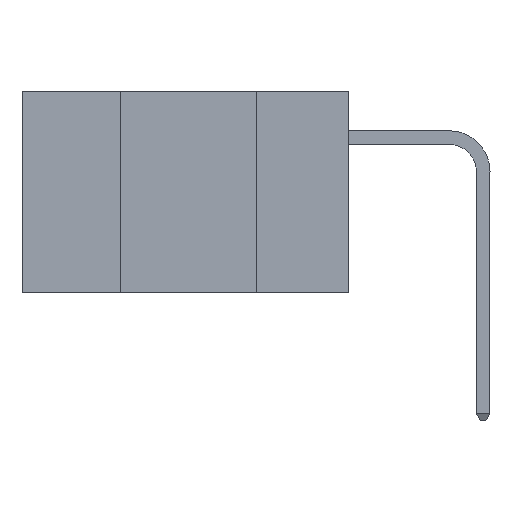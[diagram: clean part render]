
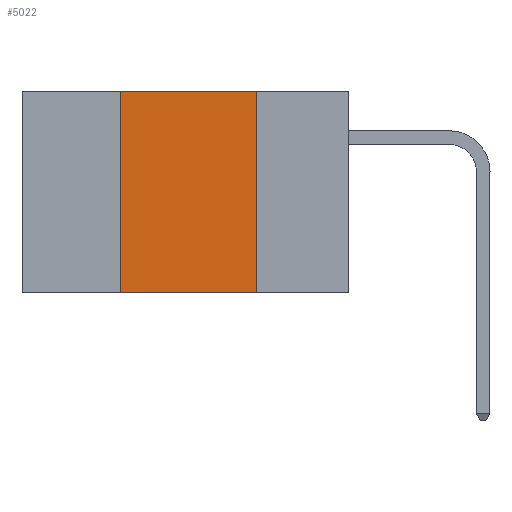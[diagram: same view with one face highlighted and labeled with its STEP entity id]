
A CAD part, left-side view. The second image highlights one B-rep face of the part: STEP entity #5022.
In plain terms, the highlighted planar face has unit normal (-1, 0, 0).
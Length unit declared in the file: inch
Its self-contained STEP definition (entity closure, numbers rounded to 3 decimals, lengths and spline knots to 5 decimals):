
#662 = ORIENTED_EDGE ( 'NONE', *, *, #5726, .F. ) ;
#873 = DIRECTION ( 'NONE',  ( 0., 0., 1. ) ) ;
#1309 = VECTOR ( 'NONE', #11218, 39.37008 ) ;
#1465 = EDGE_LOOP ( 'NONE', ( #11625, #2157, #662, #11948 ) ) ;
#1474 = CARTESIAN_POINT ( 'NONE',  ( 0., 0.42, 0. ) ) ;
#1668 = CARTESIAN_POINT ( 'NONE',  ( 0., 0.17, 0. ) ) ;
#1727 = FACE_OUTER_BOUND ( 'NONE', #1465, .T. ) ;
#2157 = ORIENTED_EDGE ( 'NONE', *, *, #7152, .F. ) ;
#2676 = DIRECTION ( 'NONE',  ( 1., 0., 0. ) ) ;
#3814 = CARTESIAN_POINT ( 'NONE',  ( 0., 0.6, -0.37 ) ) ;
#4143 = VECTOR ( 'NONE', #9492, 39.37008 ) ;
#5022 = ADVANCED_FACE ( 'NONE', ( #1727 ), #10476, .F. ) ;
#5534 = AXIS2_PLACEMENT_3D ( 'NONE', #8273, #2676, #12986 ) ;
#5726 = EDGE_CURVE ( 'NONE', #9937, #8701, #9642, .T. ) ;
#6422 = VERTEX_POINT ( 'NONE', #13944 ) ;
#7147 = VECTOR ( 'NONE', #873, 39.37008 ) ;
#7152 = EDGE_CURVE ( 'NONE', #8701, #8890, #8893, .T. ) ;
#8273 = CARTESIAN_POINT ( 'NONE',  ( 0., 0.6, 0. ) ) ;
#8697 = CARTESIAN_POINT ( 'NONE',  ( 0., 0.42, 0. ) ) ;
#8701 = VERTEX_POINT ( 'NONE', #1474 ) ;
#8890 = VERTEX_POINT ( 'NONE', #1668 ) ;
#8893 = LINE ( 'NONE', #12210, #1309 ) ;
#9318 = CARTESIAN_POINT ( 'NONE',  ( 0., 0.42, -0.37 ) ) ;
#9492 = DIRECTION ( 'NONE',  ( 0., -1., 0. ) ) ;
#9642 = LINE ( 'NONE', #8697, #7147 ) ;
#9937 = VERTEX_POINT ( 'NONE', #9318 ) ;
#10044 = CARTESIAN_POINT ( 'NONE',  ( 0., 0.17, 0. ) ) ;
#10476 = PLANE ( 'NONE',  #5534 ) ;
#10629 = LINE ( 'NONE', #3814, #4143 ) ;
#11193 = EDGE_CURVE ( 'NONE', #9937, #6422, #10629, .T. ) ;
#11218 = DIRECTION ( 'NONE',  ( 0., -1., 0. ) ) ;
#11483 = EDGE_CURVE ( 'NONE', #8890, #6422, #13387, .T. ) ;
#11625 = ORIENTED_EDGE ( 'NONE', *, *, #11483, .F. ) ;
#11671 = VECTOR ( 'NONE', #13394, 39.37008 ) ;
#11948 = ORIENTED_EDGE ( 'NONE', *, *, #11193, .T. ) ;
#12210 = CARTESIAN_POINT ( 'NONE',  ( 0., 0.6, 0. ) ) ;
#12986 = DIRECTION ( 'NONE',  ( 0., 0., -1. ) ) ;
#13387 = LINE ( 'NONE', #10044, #11671 ) ;
#13394 = DIRECTION ( 'NONE',  ( 0., 0., -1. ) ) ;
#13944 = CARTESIAN_POINT ( 'NONE',  ( 0., 0.17, -0.37 ) ) ;
